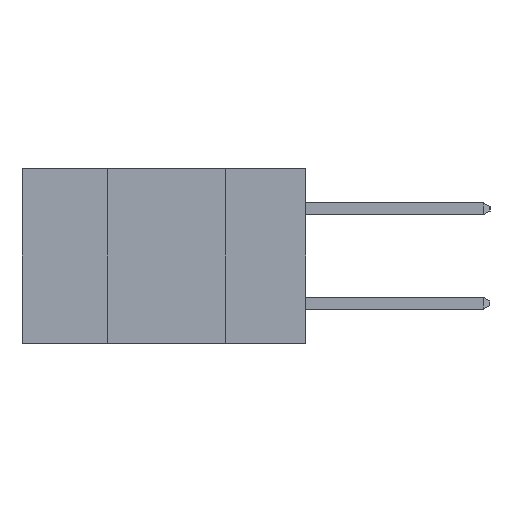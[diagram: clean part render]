
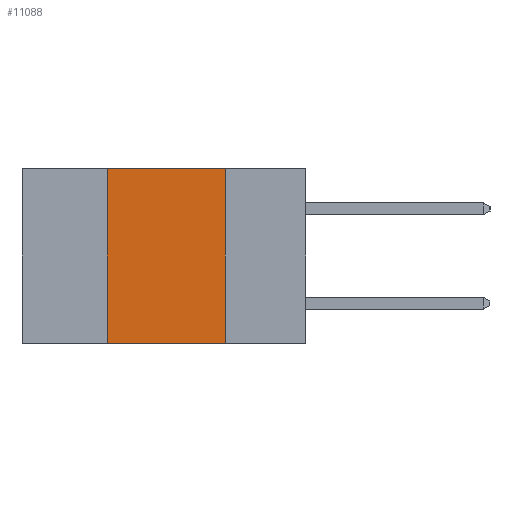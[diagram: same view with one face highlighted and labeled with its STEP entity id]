
A CAD part, left-side view. The second image highlights one B-rep face of the part: STEP entity #11088.
In plain terms, the highlighted planar face has unit normal (-1, 0, 0).
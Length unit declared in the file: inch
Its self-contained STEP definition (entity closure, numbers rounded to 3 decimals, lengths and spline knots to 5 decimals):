
#204 = VERTEX_POINT ( 'NONE', #12473 ) ;
#1016 = PLANE ( 'NONE',  #15829 ) ;
#1067 = VECTOR ( 'NONE', #7385, 39.37008 ) ;
#1310 = DIRECTION ( 'NONE',  ( 0., 0., 1. ) ) ;
#1403 = LINE ( 'NONE', #17219, #4364 ) ;
#1579 = FACE_OUTER_BOUND ( 'NONE', #3547, .T. ) ;
#1700 = CARTESIAN_POINT ( 'NONE',  ( 0., 0.42, -0.37 ) ) ;
#2224 = ORIENTED_EDGE ( 'NONE', *, *, #16324, .F. ) ;
#3547 = EDGE_LOOP ( 'NONE', ( #2224, #14618, #12532, #3749 ) ) ;
#3749 = ORIENTED_EDGE ( 'NONE', *, *, #17773, .T. ) ;
#4364 = VECTOR ( 'NONE', #12138, 39.37008 ) ;
#4689 = CARTESIAN_POINT ( 'NONE',  ( 0., 0.17, -0.37 ) ) ;
#4806 = VERTEX_POINT ( 'NONE', #1700 ) ;
#5378 = CARTESIAN_POINT ( 'NONE',  ( 0., 0.6, 0. ) ) ;
#5911 = EDGE_CURVE ( 'NONE', #15769, #204, #16421, .T. ) ;
#7385 = DIRECTION ( 'NONE',  ( 0., -1., 0. ) ) ;
#8276 = VERTEX_POINT ( 'NONE', #4689 ) ;
#8339 = CARTESIAN_POINT ( 'NONE',  ( 0., 0.42, 0. ) ) ;
#9740 = DIRECTION ( 'NONE',  ( 0., 0., -1. ) ) ;
#10174 = CARTESIAN_POINT ( 'NONE',  ( 0., 0.6, -0.37 ) ) ;
#10306 = CARTESIAN_POINT ( 'NONE',  ( 0., 0.6, 0. ) ) ;
#11088 = ADVANCED_FACE ( 'NONE', ( #1579 ), #1016, .F. ) ;
#11168 = DIRECTION ( 'NONE',  ( 0., -1., 0. ) ) ;
#11300 = CARTESIAN_POINT ( 'NONE',  ( 0., 0.42, 0. ) ) ;
#12138 = DIRECTION ( 'NONE',  ( 0., 0., -1. ) ) ;
#12473 = CARTESIAN_POINT ( 'NONE',  ( 0., 0.17, 0. ) ) ;
#12532 = ORIENTED_EDGE ( 'NONE', *, *, #17670, .F. ) ;
#13030 = VECTOR ( 'NONE', #11168, 39.37008 ) ;
#13854 = VECTOR ( 'NONE', #1310, 39.37008 ) ;
#14249 = LINE ( 'NONE', #11300, #13854 ) ;
#14618 = ORIENTED_EDGE ( 'NONE', *, *, #5911, .F. ) ;
#15430 = LINE ( 'NONE', #10174, #1067 ) ;
#15769 = VERTEX_POINT ( 'NONE', #8339 ) ;
#15829 = AXIS2_PLACEMENT_3D ( 'NONE', #5378, #17521, #9740 ) ;
#16324 = EDGE_CURVE ( 'NONE', #204, #8276, #1403, .T. ) ;
#16421 = LINE ( 'NONE', #10306, #13030 ) ;
#17219 = CARTESIAN_POINT ( 'NONE',  ( 0., 0.17, 0. ) ) ;
#17521 = DIRECTION ( 'NONE',  ( 1., 0., 0. ) ) ;
#17670 = EDGE_CURVE ( 'NONE', #4806, #15769, #14249, .T. ) ;
#17773 = EDGE_CURVE ( 'NONE', #4806, #8276, #15430, .T. ) ;
